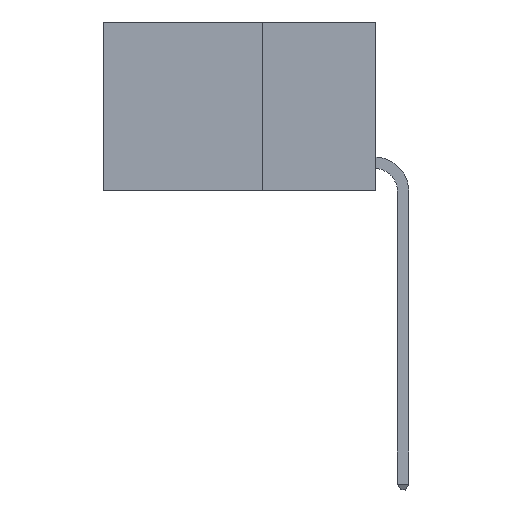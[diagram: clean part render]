
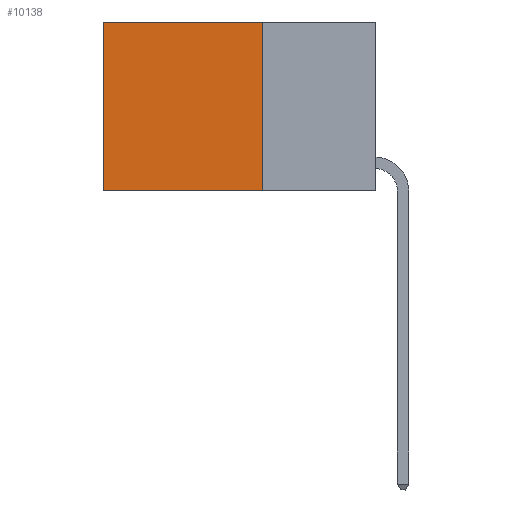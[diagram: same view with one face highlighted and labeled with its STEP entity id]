
A CAD part, left-side view. The second image highlights one B-rep face of the part: STEP entity #10138.
In plain terms, the highlighted planar face has unit normal (-1, 0, 0).
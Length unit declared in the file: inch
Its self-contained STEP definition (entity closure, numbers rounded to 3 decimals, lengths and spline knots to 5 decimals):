
#244 = EDGE_CURVE ( 'NONE', #4631, #17861, #4241, .T. ) ;
#1062 = PLANE ( 'NONE',  #16664 ) ;
#1381 = CARTESIAN_POINT ( 'NONE',  ( 0.2625, 0.25, 0. ) ) ;
#2583 = DIRECTION ( 'NONE',  ( 1., 0., 0. ) ) ;
#2951 = EDGE_CURVE ( 'NONE', #17861, #11219, #3937, .T. ) ;
#3367 = VECTOR ( 'NONE', #8028, 39.37008 ) ;
#3528 = CARTESIAN_POINT ( 'NONE',  ( 0.2625, 0.6, -0.37 ) ) ;
#3937 = LINE ( 'NONE', #14970, #11256 ) ;
#4194 = EDGE_CURVE ( 'NONE', #4631, #6167, #9848, .T. ) ;
#4241 = LINE ( 'NONE', #5010, #3367 ) ;
#4346 = ORIENTED_EDGE ( 'NONE', *, *, #5132, .F. ) ;
#4623 = DIRECTION ( 'NONE',  ( 0., 0., -1. ) ) ;
#4631 = VERTEX_POINT ( 'NONE', #1381 ) ;
#4804 = DIRECTION ( 'NONE',  ( 0., 0., -1. ) ) ;
#4957 = CARTESIAN_POINT ( 'NONE',  ( 0.2625, 0.6, 0. ) ) ;
#5010 = CARTESIAN_POINT ( 'NONE',  ( 0.2625, 0.25, 0. ) ) ;
#5132 = EDGE_CURVE ( 'NONE', #6167, #11219, #17470, .T. ) ;
#5931 = ORIENTED_EDGE ( 'NONE', *, *, #4194, .F. ) ;
#6167 = VERTEX_POINT ( 'NONE', #7131 ) ;
#7131 = CARTESIAN_POINT ( 'NONE',  ( 0.2625, 0.25, -0.37 ) ) ;
#8028 = DIRECTION ( 'NONE',  ( 0., 1., 0. ) ) ;
#9848 = LINE ( 'NONE', #14797, #10292 ) ;
#10138 = ADVANCED_FACE ( 'NONE', ( #18772 ), #1062, .F. ) ;
#10292 = VECTOR ( 'NONE', #4623, 39.37008 ) ;
#11219 = VERTEX_POINT ( 'NONE', #3528 ) ;
#11256 = VECTOR ( 'NONE', #4804, 39.37008 ) ;
#11826 = EDGE_LOOP ( 'NONE', ( #15381, #4346, #5931, #15594 ) ) ;
#12777 = DIRECTION ( 'NONE',  ( 0., 0., -1. ) ) ;
#14797 = CARTESIAN_POINT ( 'NONE',  ( 0.2625, 0.25, 0. ) ) ;
#14970 = CARTESIAN_POINT ( 'NONE',  ( 0.2625, 0.6, 0. ) ) ;
#15381 = ORIENTED_EDGE ( 'NONE', *, *, #2951, .T. ) ;
#15581 = CARTESIAN_POINT ( 'NONE',  ( 0.2625, 0.25, -0.37 ) ) ;
#15594 = ORIENTED_EDGE ( 'NONE', *, *, #244, .T. ) ;
#16664 = AXIS2_PLACEMENT_3D ( 'NONE', #18472, #2583, #12777 ) ;
#17006 = DIRECTION ( 'NONE',  ( 0., 1., 0. ) ) ;
#17470 = LINE ( 'NONE', #15581, #18350 ) ;
#17861 = VERTEX_POINT ( 'NONE', #4957 ) ;
#18350 = VECTOR ( 'NONE', #17006, 39.37008 ) ;
#18472 = CARTESIAN_POINT ( 'NONE',  ( 0.2625, 0.25, 0. ) ) ;
#18772 = FACE_OUTER_BOUND ( 'NONE', #11826, .T. ) ;
